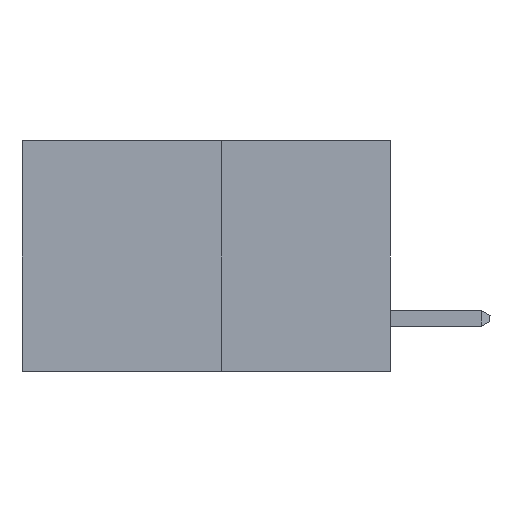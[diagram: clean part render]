
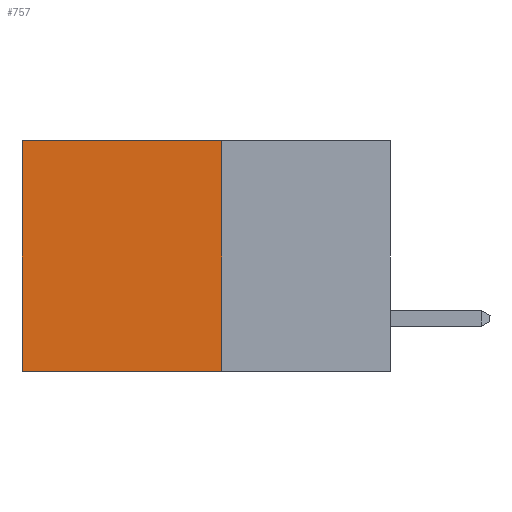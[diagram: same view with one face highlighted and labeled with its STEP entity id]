
A CAD part, left-side view. The second image highlights one B-rep face of the part: STEP entity #757.
In plain terms, the highlighted planar face has unit normal (-1, 0, 0).
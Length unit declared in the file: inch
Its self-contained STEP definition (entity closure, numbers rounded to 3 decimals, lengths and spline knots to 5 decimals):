
#647 = LINE ( 'NONE', #1700, #5759 ) ;
#730 = VECTOR ( 'NONE', #16188, 39.37008 ) ;
#757 = ADVANCED_FACE ( 'NONE', ( #26802 ), #11317, .F. ) ;
#1700 = CARTESIAN_POINT ( 'NONE',  ( 0.277, 0.27, -0.37 ) ) ;
#4767 = DIRECTION ( 'NONE',  ( 1., 0., 0. ) ) ;
#5480 = EDGE_CURVE ( 'NONE', #13191, #27869, #647, .T. ) ;
#5759 = VECTOR ( 'NONE', #15487, 39.37008 ) ;
#5852 = LINE ( 'NONE', #22792, #730 ) ;
#7840 = VERTEX_POINT ( 'NONE', #12536 ) ;
#8369 = ORIENTED_EDGE ( 'NONE', *, *, #25841, .T. ) ;
#8416 = LINE ( 'NONE', #17013, #19258 ) ;
#9082 = DIRECTION ( 'NONE',  ( 0., 0., -1. ) ) ;
#9924 = ORIENTED_EDGE ( 'NONE', *, *, #17347, .T. ) ;
#11317 = PLANE ( 'NONE',  #24487 ) ;
#11840 = VERTEX_POINT ( 'NONE', #20501 ) ;
#12536 = CARTESIAN_POINT ( 'NONE',  ( 0.277, 0.59, 0. ) ) ;
#13191 = VERTEX_POINT ( 'NONE', #24908 ) ;
#13733 = ORIENTED_EDGE ( 'NONE', *, *, #20905, .F. ) ;
#15487 = DIRECTION ( 'NONE',  ( 0., 1., 0. ) ) ;
#16188 = DIRECTION ( 'NONE',  ( 0., 0., -1. ) ) ;
#17013 = CARTESIAN_POINT ( 'NONE',  ( 0.277, 0.27, 0. ) ) ;
#17347 = EDGE_CURVE ( 'NONE', #11840, #7840, #8416, .T. ) ;
#17743 = CARTESIAN_POINT ( 'NONE',  ( 0.277, 0.27, -0.37 ) ) ;
#17907 = VECTOR ( 'NONE', #9082, 39.37008 ) ;
#18007 = ORIENTED_EDGE ( 'NONE', *, *, #5480, .F. ) ;
#18059 = CARTESIAN_POINT ( 'NONE',  ( 0.277, 0.59, -0.37 ) ) ;
#19258 = VECTOR ( 'NONE', #21734, 39.37008 ) ;
#19871 = CARTESIAN_POINT ( 'NONE',  ( 0.277, 0.59, -0.37 ) ) ;
#19952 = DIRECTION ( 'NONE',  ( 0., 0., -1. ) ) ;
#20501 = CARTESIAN_POINT ( 'NONE',  ( 0.277, 0.27, 0. ) ) ;
#20905 = EDGE_CURVE ( 'NONE', #11840, #13191, #5852, .T. ) ;
#21734 = DIRECTION ( 'NONE',  ( 0., 1., 0. ) ) ;
#22330 = EDGE_LOOP ( 'NONE', ( #8369, #18007, #13733, #9924 ) ) ;
#22792 = CARTESIAN_POINT ( 'NONE',  ( 0.277, 0.27, -0.37 ) ) ;
#24385 = LINE ( 'NONE', #19871, #17907 ) ;
#24487 = AXIS2_PLACEMENT_3D ( 'NONE', #17743, #4767, #19952 ) ;
#24908 = CARTESIAN_POINT ( 'NONE',  ( 0.277, 0.27, -0.37 ) ) ;
#25841 = EDGE_CURVE ( 'NONE', #7840, #27869, #24385, .T. ) ;
#26802 = FACE_OUTER_BOUND ( 'NONE', #22330, .T. ) ;
#27869 = VERTEX_POINT ( 'NONE', #18059 ) ;
